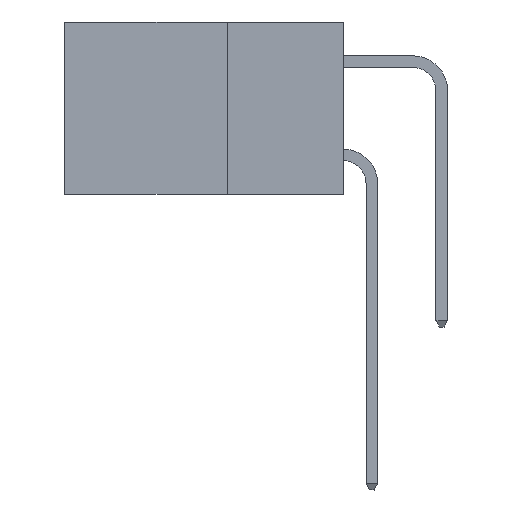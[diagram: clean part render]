
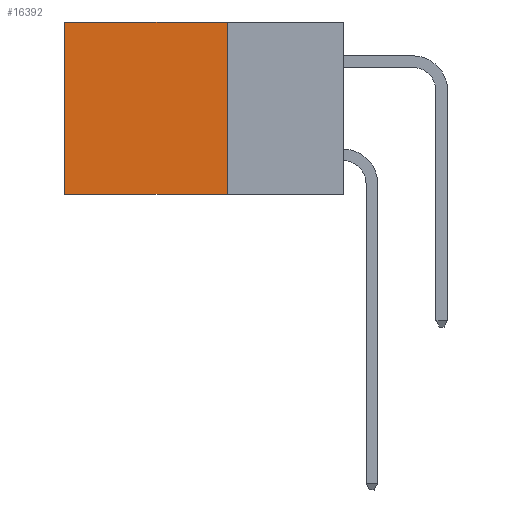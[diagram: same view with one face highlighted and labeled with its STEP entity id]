
A CAD part, left-side view. The second image highlights one B-rep face of the part: STEP entity #16392.
In plain terms, the highlighted planar face has unit normal (-1, 0, 0).
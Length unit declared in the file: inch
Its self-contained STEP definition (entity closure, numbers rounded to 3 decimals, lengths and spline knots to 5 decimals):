
#87 = EDGE_CURVE ( 'NONE', #9160, #13675, #7889, .T. ) ;
#98 = VECTOR ( 'NONE', #3336, 39.37008 ) ;
#181 = CARTESIAN_POINT ( 'NONE',  ( 0.298, 0.6, 0. ) ) ;
#682 = VERTEX_POINT ( 'NONE', #4867 ) ;
#1705 = CARTESIAN_POINT ( 'NONE',  ( 0.298, 0.6, 0. ) ) ;
#1837 = CARTESIAN_POINT ( 'NONE',  ( 0.298, 0.25, -0.37 ) ) ;
#2087 = EDGE_CURVE ( 'NONE', #10529, #682, #15060, .T. ) ;
#2370 = ORIENTED_EDGE ( 'NONE', *, *, #87, .T. ) ;
#3336 = DIRECTION ( 'NONE',  ( 0., 1., 0. ) ) ;
#3946 = PLANE ( 'NONE',  #8899 ) ;
#3999 = CARTESIAN_POINT ( 'NONE',  ( 0.298, 0.25, 0. ) ) ;
#4140 = VECTOR ( 'NONE', #12676, 39.37008 ) ;
#4167 = LINE ( 'NONE', #181, #7462 ) ;
#4241 = DIRECTION ( 'NONE',  ( 0., 0., -1. ) ) ;
#4867 = CARTESIAN_POINT ( 'NONE',  ( 0.298, 0.6, -0.37 ) ) ;
#4974 = CARTESIAN_POINT ( 'NONE',  ( 0.298, 0.25, 0. ) ) ;
#5405 = DIRECTION ( 'NONE',  ( 0., 0., -1. ) ) ;
#5427 = ORIENTED_EDGE ( 'NONE', *, *, #2087, .F. ) ;
#6707 = EDGE_CURVE ( 'NONE', #9160, #10529, #7189, .T. ) ;
#7189 = LINE ( 'NONE', #4974, #10436 ) ;
#7457 = CARTESIAN_POINT ( 'NONE',  ( 0.298, 0.25, 0. ) ) ;
#7462 = VECTOR ( 'NONE', #4241, 39.37008 ) ;
#7889 = LINE ( 'NONE', #7457, #4140 ) ;
#8899 = AXIS2_PLACEMENT_3D ( 'NONE', #3999, #13796, #5405 ) ;
#9160 = VERTEX_POINT ( 'NONE', #15536 ) ;
#9574 = ORIENTED_EDGE ( 'NONE', *, *, #11023, .T. ) ;
#10436 = VECTOR ( 'NONE', #17591, 39.37008 ) ;
#10529 = VERTEX_POINT ( 'NONE', #15786 ) ;
#11023 = EDGE_CURVE ( 'NONE', #13675, #682, #4167, .T. ) ;
#11355 = EDGE_LOOP ( 'NONE', ( #9574, #5427, #17759, #2370 ) ) ;
#11653 = FACE_OUTER_BOUND ( 'NONE', #11355, .T. ) ;
#12676 = DIRECTION ( 'NONE',  ( 0., 1., 0. ) ) ;
#13675 = VERTEX_POINT ( 'NONE', #1705 ) ;
#13796 = DIRECTION ( 'NONE',  ( 1., 0., 0. ) ) ;
#15060 = LINE ( 'NONE', #1837, #98 ) ;
#15536 = CARTESIAN_POINT ( 'NONE',  ( 0.298, 0.25, 0. ) ) ;
#15786 = CARTESIAN_POINT ( 'NONE',  ( 0.298, 0.25, -0.37 ) ) ;
#16392 = ADVANCED_FACE ( 'NONE', ( #11653 ), #3946, .F. ) ;
#17591 = DIRECTION ( 'NONE',  ( 0., 0., -1. ) ) ;
#17759 = ORIENTED_EDGE ( 'NONE', *, *, #6707, .F. ) ;
